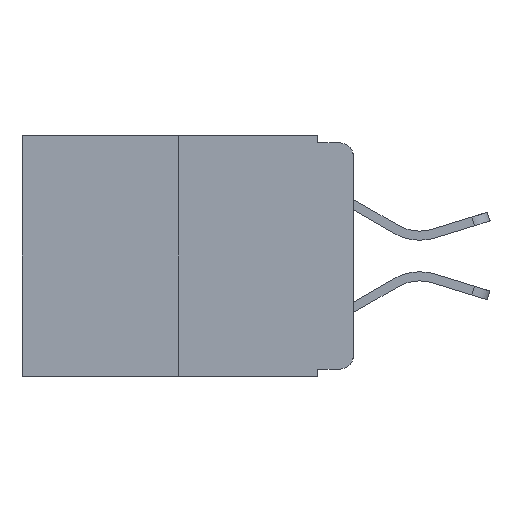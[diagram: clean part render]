
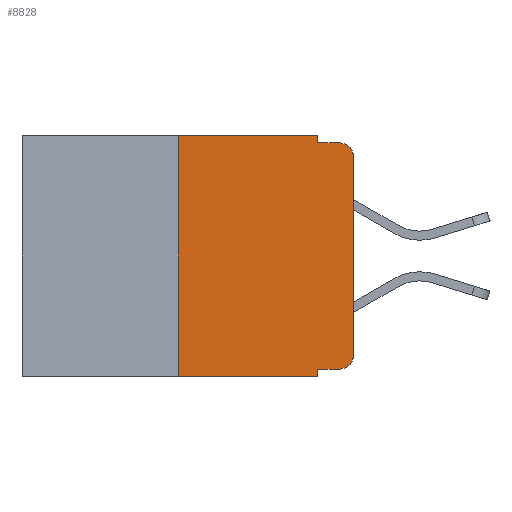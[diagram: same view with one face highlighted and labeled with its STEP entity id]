
A CAD part, left-side view. The second image highlights one B-rep face of the part: STEP entity #8828.
In plain terms, the highlighted planar face has unit normal (-1, 0, 0).
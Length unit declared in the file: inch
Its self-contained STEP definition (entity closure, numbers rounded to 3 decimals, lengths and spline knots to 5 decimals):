
#98 = CIRCLE ( 'NONE', #18836, 0.02 ) ;
#131 = DIRECTION ( 'NONE',  ( 0., 0., -1. ) ) ;
#172 = DIRECTION ( 'NONE',  ( 0., -1., 0. ) ) ;
#280 = EDGE_CURVE ( 'NONE', #8283, #22443, #15316, .T. ) ;
#935 = EDGE_LOOP ( 'NONE', ( #11291, #11845, #20925, #2472, #12985, #8772, #9315, #18601, #9867, #19645 ) ) ;
#1096 = VECTOR ( 'NONE', #9391, 39.37008 ) ;
#1224 = CARTESIAN_POINT ( 'NONE',  ( 0., 0.473, -0.343 ) ) ;
#1885 = VERTEX_POINT ( 'NONE', #12231 ) ;
#2095 = CARTESIAN_POINT ( 'NONE',  ( 0., 0.473, 0. ) ) ;
#2472 = ORIENTED_EDGE ( 'NONE', *, *, #280, .F. ) ;
#2526 = VECTOR ( 'NONE', #2653, 39.37008 ) ;
#2653 = DIRECTION ( 'NONE',  ( 0., 0., -1. ) ) ;
#3328 = EDGE_CURVE ( 'NONE', #1885, #6595, #17041, .T. ) ;
#3951 = DIRECTION ( 'NONE',  ( 0., -1., 0. ) ) ;
#4312 = CARTESIAN_POINT ( 'NONE',  ( 0., 0.02, -0.333 ) ) ;
#4358 = CARTESIAN_POINT ( 'NONE',  ( 0., 0.051, 0. ) ) ;
#4533 = LINE ( 'NONE', #16588, #14256 ) ;
#4671 = EDGE_CURVE ( 'NONE', #15303, #6595, #16210, .T. ) ;
#5031 = DIRECTION ( 'NONE',  ( -1., 0., 0. ) ) ;
#5172 = VECTOR ( 'NONE', #15300, 39.37008 ) ;
#5744 = EDGE_CURVE ( 'NONE', #11554, #6039, #6371, .T. ) ;
#5884 = EDGE_CURVE ( 'NONE', #10409, #8283, #8406, .T. ) ;
#6039 = VERTEX_POINT ( 'NONE', #14321 ) ;
#6371 = LINE ( 'NONE', #21369, #1096 ) ;
#6595 = VERTEX_POINT ( 'NONE', #10650 ) ;
#7255 = EDGE_CURVE ( 'NONE', #6039, #22705, #17848, .T. ) ;
#7300 = VECTOR ( 'NONE', #172, 39.37008 ) ;
#7838 = AXIS2_PLACEMENT_3D ( 'NONE', #20012, #9632, #21666 ) ;
#8114 = VERTEX_POINT ( 'NONE', #4312 ) ;
#8283 = VERTEX_POINT ( 'NONE', #18982 ) ;
#8309 = CARTESIAN_POINT ( 'NONE',  ( 0., 0.02, -0.01 ) ) ;
#8406 = LINE ( 'NONE', #21854, #7300 ) ;
#8772 = ORIENTED_EDGE ( 'NONE', *, *, #14361, .F. ) ;
#8828 = ADVANCED_FACE ( 'NONE', ( #19380 ), #9812, .F. ) ;
#9315 = ORIENTED_EDGE ( 'NONE', *, *, #4671, .T. ) ;
#9391 = DIRECTION ( 'NONE',  ( 0., 0., 1. ) ) ;
#9632 = DIRECTION ( 'NONE',  ( -1., 0., 0. ) ) ;
#9750 = EDGE_CURVE ( 'NONE', #8114, #11554, #98, .T. ) ;
#9812 = PLANE ( 'NONE',  #11582 ) ;
#9867 = ORIENTED_EDGE ( 'NONE', *, *, #18252, .T. ) ;
#10079 = LINE ( 'NONE', #21937, #5172 ) ;
#10409 = VERTEX_POINT ( 'NONE', #17580 ) ;
#10650 = CARTESIAN_POINT ( 'NONE',  ( 0., 0.051, -0.343 ) ) ;
#11291 = ORIENTED_EDGE ( 'NONE', *, *, #5744, .T. ) ;
#11554 = VERTEX_POINT ( 'NONE', #14894 ) ;
#11582 = AXIS2_PLACEMENT_3D ( 'NONE', #2095, #11633, #131 ) ;
#11633 = DIRECTION ( 'NONE',  ( 1., 0., 0. ) ) ;
#11742 = DIRECTION ( 'NONE',  ( 0., 0., -1. ) ) ;
#11845 = ORIENTED_EDGE ( 'NONE', *, *, #7255, .T. ) ;
#12231 = CARTESIAN_POINT ( 'NONE',  ( 0., 0.051, -0.333 ) ) ;
#12985 = ORIENTED_EDGE ( 'NONE', *, *, #5884, .F. ) ;
#13549 = CARTESIAN_POINT ( 'NONE',  ( 0., 0.051, 0. ) ) ;
#14256 = VECTOR ( 'NONE', #3951, 39.37008 ) ;
#14319 = DIRECTION ( 'NONE',  ( 0., -1., 0. ) ) ;
#14321 = CARTESIAN_POINT ( 'NONE',  ( 0., 0., -0.03 ) ) ;
#14361 = EDGE_CURVE ( 'NONE', #15303, #10409, #10079, .T. ) ;
#14790 = CARTESIAN_POINT ( 'NONE',  ( 0., 0.051, -0.01 ) ) ;
#14894 = CARTESIAN_POINT ( 'NONE',  ( 0., 0., -0.313 ) ) ;
#15300 = DIRECTION ( 'NONE',  ( 0., 0., 1. ) ) ;
#15303 = VERTEX_POINT ( 'NONE', #22590 ) ;
#15316 = LINE ( 'NONE', #13549, #19283 ) ;
#15567 = EDGE_CURVE ( 'NONE', #22443, #22705, #4533, .T. ) ;
#15847 = CARTESIAN_POINT ( 'NONE',  ( 0., 0.02, -0.313 ) ) ;
#16210 = LINE ( 'NONE', #1224, #21181 ) ;
#16588 = CARTESIAN_POINT ( 'NONE',  ( 0., 0.051, -0.01 ) ) ;
#17041 = LINE ( 'NONE', #4358, #2526 ) ;
#17514 = DIRECTION ( 'NONE',  ( 0., 0., -1. ) ) ;
#17580 = CARTESIAN_POINT ( 'NONE',  ( 0., 0.25, 0. ) ) ;
#17848 = CIRCLE ( 'NONE', #7838, 0.02 ) ;
#17867 = LINE ( 'NONE', #18986, #19698 ) ;
#18252 = EDGE_CURVE ( 'NONE', #1885, #8114, #17867, .T. ) ;
#18601 = ORIENTED_EDGE ( 'NONE', *, *, #3328, .F. ) ;
#18836 = AXIS2_PLACEMENT_3D ( 'NONE', #15847, #5031, #17514 ) ;
#18914 = DIRECTION ( 'NONE',  ( 0., -1., 0. ) ) ;
#18982 = CARTESIAN_POINT ( 'NONE',  ( 0., 0.051, 0. ) ) ;
#18986 = CARTESIAN_POINT ( 'NONE',  ( 0., 0.051, -0.333 ) ) ;
#19283 = VECTOR ( 'NONE', #11742, 39.37008 ) ;
#19380 = FACE_OUTER_BOUND ( 'NONE', #935, .T. ) ;
#19645 = ORIENTED_EDGE ( 'NONE', *, *, #9750, .T. ) ;
#19698 = VECTOR ( 'NONE', #18914, 39.37008 ) ;
#20012 = CARTESIAN_POINT ( 'NONE',  ( 0., 0.02, -0.03 ) ) ;
#20925 = ORIENTED_EDGE ( 'NONE', *, *, #15567, .F. ) ;
#21181 = VECTOR ( 'NONE', #14319, 39.37008 ) ;
#21369 = CARTESIAN_POINT ( 'NONE',  ( 0., 0., 0. ) ) ;
#21666 = DIRECTION ( 'NONE',  ( 0., 0., -1. ) ) ;
#21854 = CARTESIAN_POINT ( 'NONE',  ( 0., 0.473, 0. ) ) ;
#21937 = CARTESIAN_POINT ( 'NONE',  ( 0., 0.25, 0. ) ) ;
#22443 = VERTEX_POINT ( 'NONE', #14790 ) ;
#22590 = CARTESIAN_POINT ( 'NONE',  ( 0., 0.25, -0.343 ) ) ;
#22705 = VERTEX_POINT ( 'NONE', #8309 ) ;
